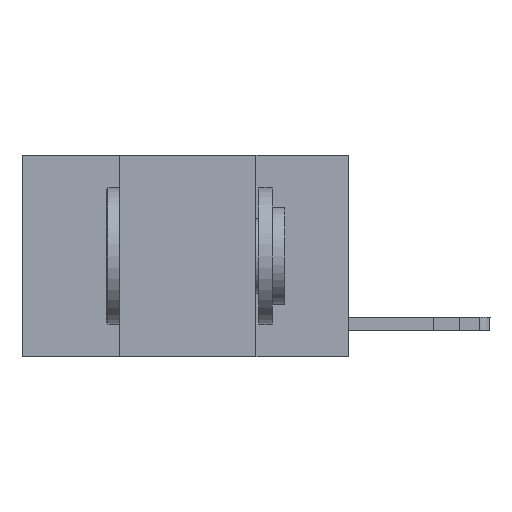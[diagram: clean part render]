
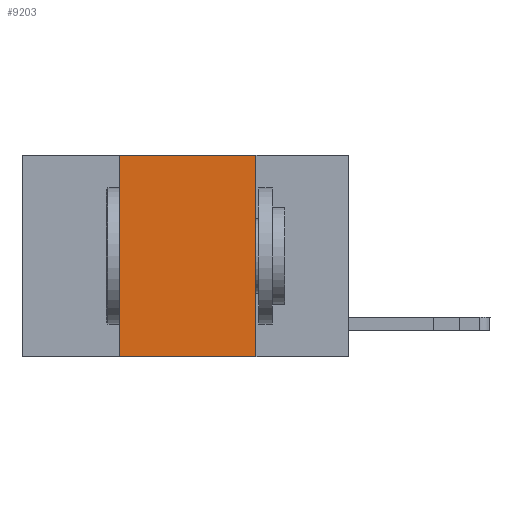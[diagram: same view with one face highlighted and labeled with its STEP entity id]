
A CAD part, left-side view. The second image highlights one B-rep face of the part: STEP entity #9203.
In plain terms, the highlighted planar face has unit normal (-1, 0, 0).
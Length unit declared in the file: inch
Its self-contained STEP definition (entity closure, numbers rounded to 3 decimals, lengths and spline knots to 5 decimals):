
#363 = VERTEX_POINT ( 'NONE', #11500 ) ;
#650 = EDGE_CURVE ( 'NONE', #363, #11031, #5148, .T. ) ;
#730 = DIRECTION ( 'NONE',  ( 0., -1., 0. ) ) ;
#794 = LINE ( 'NONE', #9692, #15983 ) ;
#946 = CARTESIAN_POINT ( 'NONE',  ( 0., 0.6, 0. ) ) ;
#1484 = LINE ( 'NONE', #18045, #12753 ) ;
#1775 = EDGE_CURVE ( 'NONE', #12397, #10176, #1484, .T. ) ;
#2414 = DIRECTION ( 'NONE',  ( 0., 0., -1. ) ) ;
#3150 = ORIENTED_EDGE ( 'NONE', *, *, #650, .F. ) ;
#4108 = DIRECTION ( 'NONE',  ( 0., 0., -1. ) ) ;
#5110 = CARTESIAN_POINT ( 'NONE',  ( 0., 0.42, 0. ) ) ;
#5148 = LINE ( 'NONE', #15383, #8122 ) ;
#5797 = FACE_OUTER_BOUND ( 'NONE', #17249, .T. ) ;
#7077 = EDGE_CURVE ( 'NONE', #363, #10176, #794, .T. ) ;
#7636 = VECTOR ( 'NONE', #730, 39.37008 ) ;
#8019 = CARTESIAN_POINT ( 'NONE',  ( 0., 0.6, 0. ) ) ;
#8122 = VECTOR ( 'NONE', #10662, 39.37008 ) ;
#8206 = EDGE_CURVE ( 'NONE', #11031, #12397, #12033, .T. ) ;
#8904 = CARTESIAN_POINT ( 'NONE',  ( 0., 0.17, -0.37 ) ) ;
#9203 = ADVANCED_FACE ( 'NONE', ( #5797 ), #14135, .F. ) ;
#9692 = CARTESIAN_POINT ( 'NONE',  ( 0., 0.6, -0.37 ) ) ;
#10154 = CARTESIAN_POINT ( 'NONE',  ( 0., 0.17, 0. ) ) ;
#10176 = VERTEX_POINT ( 'NONE', #8904 ) ;
#10662 = DIRECTION ( 'NONE',  ( 0., 0., 1. ) ) ;
#11031 = VERTEX_POINT ( 'NONE', #5110 ) ;
#11171 = DIRECTION ( 'NONE',  ( 0., -1., 0. ) ) ;
#11219 = DIRECTION ( 'NONE',  ( 1., 0., 0. ) ) ;
#11500 = CARTESIAN_POINT ( 'NONE',  ( 0., 0.42, -0.37 ) ) ;
#12033 = LINE ( 'NONE', #8019, #7636 ) ;
#12397 = VERTEX_POINT ( 'NONE', #10154 ) ;
#12753 = VECTOR ( 'NONE', #4108, 39.37008 ) ;
#14135 = PLANE ( 'NONE',  #17610 ) ;
#15383 = CARTESIAN_POINT ( 'NONE',  ( 0., 0.42, 0. ) ) ;
#15853 = ORIENTED_EDGE ( 'NONE', *, *, #7077, .T. ) ;
#15983 = VECTOR ( 'NONE', #11171, 39.37008 ) ;
#16252 = ORIENTED_EDGE ( 'NONE', *, *, #1775, .F. ) ;
#17249 = EDGE_LOOP ( 'NONE', ( #16252, #17295, #3150, #15853 ) ) ;
#17295 = ORIENTED_EDGE ( 'NONE', *, *, #8206, .F. ) ;
#17610 = AXIS2_PLACEMENT_3D ( 'NONE', #946, #11219, #2414 ) ;
#18045 = CARTESIAN_POINT ( 'NONE',  ( 0., 0.17, 0. ) ) ;
